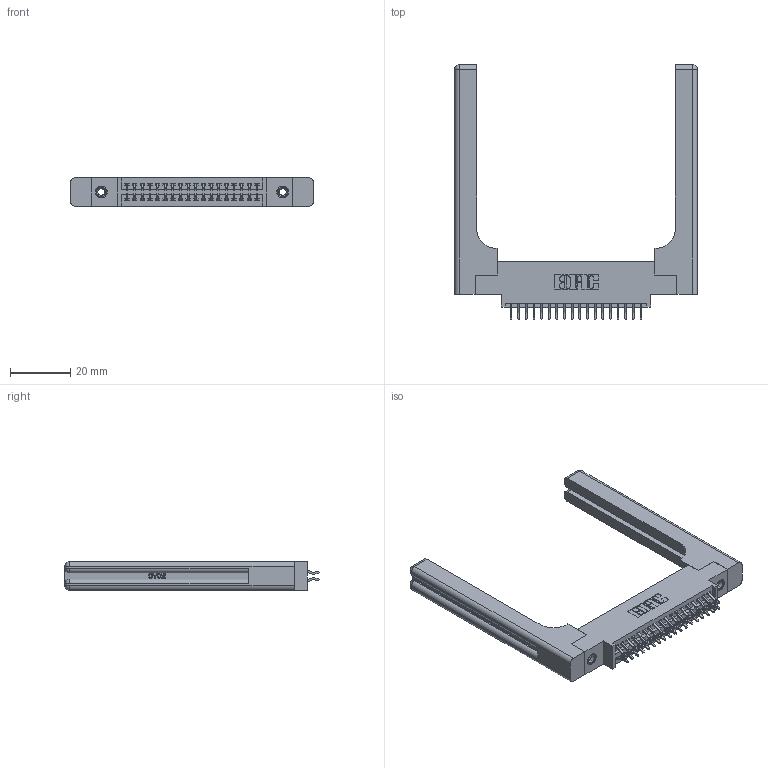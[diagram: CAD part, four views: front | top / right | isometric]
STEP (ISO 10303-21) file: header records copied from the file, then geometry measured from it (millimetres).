
FILE_DESCRIPTION (( 'STEP AP203' ), '1' );
FILE_NAME ('395-036-556-858.STEP', '2019-10-18T02:54:13', ( '' ), ( '' ), 'SwSTEP 2.0', 'SolidWorks 2016', '' );
FILE_SCHEMA (( 'CONFIG_CONTROL_DESIGN' ));
Length unit declared in the file: inch
Products named in the file (5): 345 Part_0.170 Offset - 0.156 Dia-TH; 345-292-001_556 Tail; 345-250-001_345-250-001-102; 345-220-058_345-220-058; 395-036-556-858
Assembly tree (41 placements, depth 2):
  395-036-556-858
    345 Part_0.170 Offset - 0.156 Dia-TH
    345-292-001_556 Tail  x36
    345-250-001_345-250-001-102  x2
    345-220-058_345-220-058  x2
Bounding box: 80.75 x 84.51 x 9.4 mm (x, y, z)
Volume: 15981.3 mm3; surface area: 15801.5 mm2
Topology: 41 solids, 41 shells, 2402 faces, 7031 edges, 4618 vertices
Faces by surface type: plane 1564, cylinder 778, bspline 36, cone 12, sphere 8, torus 4
Entity records: 22888 total; most frequent: CARTESIAN_POINT 4869, ORIENTED_EDGE 3588, DIRECTION 3242, EDGE_CURVE 1794, LINE 1490, VECTOR 1490, VERTEX_POINT 1186, AXIS2_PLACEMENT_3D 876
